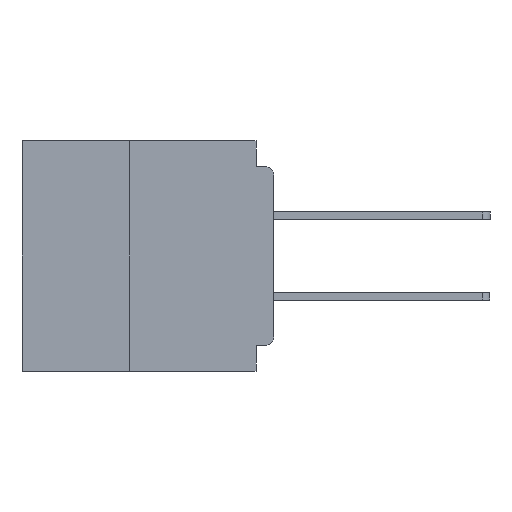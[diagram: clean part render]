
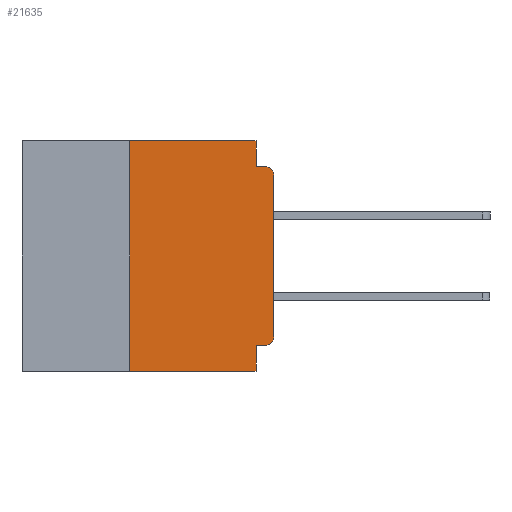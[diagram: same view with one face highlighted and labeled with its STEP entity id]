
A CAD part, left-side view. The second image highlights one B-rep face of the part: STEP entity #21635.
In plain terms, the highlighted planar face has unit normal (-1, 0, 0).
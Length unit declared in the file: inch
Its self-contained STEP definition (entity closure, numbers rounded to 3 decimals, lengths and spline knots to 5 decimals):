
#830 = CARTESIAN_POINT ( 'NONE',  ( 0., 0.031, 0. ) ) ;
#1980 = VECTOR ( 'NONE', #3878, 39.37008 ) ;
#3094 = ORIENTED_EDGE ( 'NONE', *, *, #14079, .T. ) ;
#3590 = DIRECTION ( 'NONE',  ( 0., -1., 0. ) ) ;
#3734 = VERTEX_POINT ( 'NONE', #43032 ) ;
#3878 = DIRECTION ( 'NONE',  ( 0., 0., 1. ) ) ;
#4229 = DIRECTION ( 'NONE',  ( 0., 0., -1. ) ) ;
#4340 = EDGE_LOOP ( 'NONE', ( #55539, #3094, #24114, #28395, #24261, #17673, #42425, #22083, #47247, #50970 ) ) ;
#7259 = VECTOR ( 'NONE', #3590, 39.37008 ) ;
#10152 = VERTEX_POINT ( 'NONE', #34538 ) ;
#10997 = LINE ( 'NONE', #52214, #56414 ) ;
#12163 = CARTESIAN_POINT ( 'NONE',  ( 0., 0.437, 0. ) ) ;
#13002 = VERTEX_POINT ( 'NONE', #40879 ) ;
#14079 = EDGE_CURVE ( 'NONE', #30475, #32978, #47007, .T. ) ;
#14602 = DIRECTION ( 'NONE',  ( 0., -1., 0. ) ) ;
#14851 = DIRECTION ( 'NONE',  ( 0., 0., -1. ) ) ;
#15622 = VECTOR ( 'NONE', #14602, 39.37008 ) ;
#15661 = DIRECTION ( 'NONE',  ( 0., 1., 0. ) ) ;
#15958 = EDGE_CURVE ( 'NONE', #10152, #30475, #38925, .T. ) ;
#17104 = VERTEX_POINT ( 'NONE', #26085 ) ;
#17262 = CARTESIAN_POINT ( 'NONE',  ( 0., 0., 0. ) ) ;
#17273 = DIRECTION ( 'NONE',  ( 0., 0., -1. ) ) ;
#17673 = ORIENTED_EDGE ( 'NONE', *, *, #23747, .F. ) ;
#17757 = EDGE_CURVE ( 'NONE', #3734, #13002, #10997, .T. ) ;
#19141 = CARTESIAN_POINT ( 'NONE',  ( 0., 0.437, -0.4 ) ) ;
#19378 = VERTEX_POINT ( 'NONE', #44471 ) ;
#20764 = EDGE_CURVE ( 'NONE', #30502, #13002, #28843, .T. ) ;
#21127 = VERTEX_POINT ( 'NONE', #43702 ) ;
#21635 = ADVANCED_FACE ( 'NONE', ( #37666 ), #57105, .F. ) ;
#22083 = ORIENTED_EDGE ( 'NONE', *, *, #17757, .F. ) ;
#22305 = CARTESIAN_POINT ( 'NONE',  ( 0., 0.25, -0.4 ) ) ;
#22745 = CARTESIAN_POINT ( 'NONE',  ( 0., 0.015, -0.34 ) ) ;
#23036 = VECTOR ( 'NONE', #38690, 39.37008 ) ;
#23747 = EDGE_CURVE ( 'NONE', #30502, #17104, #49830, .T. ) ;
#23801 = AXIS2_PLACEMENT_3D ( 'NONE', #22745, #53344, #27185 ) ;
#24005 = LINE ( 'NONE', #50662, #45956 ) ;
#24114 = ORIENTED_EDGE ( 'NONE', *, *, #49516, .F. ) ;
#24261 = ORIENTED_EDGE ( 'NONE', *, *, #52717, .F. ) ;
#25571 = AXIS2_PLACEMENT_3D ( 'NONE', #26553, #57095, #30978 ) ;
#25945 = CARTESIAN_POINT ( 'NONE',  ( 0., 0., -0.045 ) ) ;
#26085 = CARTESIAN_POINT ( 'NONE',  ( 0., 0.25, 0. ) ) ;
#26538 = VECTOR ( 'NONE', #40955, 39.37008 ) ;
#26553 = CARTESIAN_POINT ( 'NONE',  ( 0., 0.015, -0.06 ) ) ;
#27185 = DIRECTION ( 'NONE',  ( 0., 0., -1. ) ) ;
#28105 = CARTESIAN_POINT ( 'NONE',  ( 0., 0.031, 0. ) ) ;
#28395 = ORIENTED_EDGE ( 'NONE', *, *, #38484, .F. ) ;
#28843 = LINE ( 'NONE', #19141, #15622 ) ;
#28996 = EDGE_CURVE ( 'NONE', #19378, #3734, #24005, .T. ) ;
#29566 = LINE ( 'NONE', #25945, #7259 ) ;
#30475 = VERTEX_POINT ( 'NONE', #35217 ) ;
#30502 = VERTEX_POINT ( 'NONE', #22305 ) ;
#30524 = CARTESIAN_POINT ( 'NONE',  ( 0., 0.015, -0.045 ) ) ;
#30978 = DIRECTION ( 'NONE',  ( 0., 0., -1. ) ) ;
#30983 = DIRECTION ( 'NONE',  ( 1., 0., 0. ) ) ;
#31220 = CIRCLE ( 'NONE', #23801, 0.015 ) ;
#32068 = VECTOR ( 'NONE', #14851, 39.37008 ) ;
#32978 = VERTEX_POINT ( 'NONE', #30524 ) ;
#33473 = LINE ( 'NONE', #28105, #32068 ) ;
#34538 = CARTESIAN_POINT ( 'NONE',  ( 0., 0., -0.34 ) ) ;
#34750 = LINE ( 'NONE', #12163, #23036 ) ;
#35032 = CARTESIAN_POINT ( 'NONE',  ( 0., 0.437, 0. ) ) ;
#35217 = CARTESIAN_POINT ( 'NONE',  ( 0., 0., -0.06 ) ) ;
#36554 = CARTESIAN_POINT ( 'NONE',  ( 0., 0.25, -0.4 ) ) ;
#37666 = FACE_OUTER_BOUND ( 'NONE', #4340, .T. ) ;
#38484 = EDGE_CURVE ( 'NONE', #55324, #21127, #33473, .T. ) ;
#38690 = DIRECTION ( 'NONE',  ( 0., -1., 0. ) ) ;
#38925 = LINE ( 'NONE', #17262, #1980 ) ;
#40879 = CARTESIAN_POINT ( 'NONE',  ( 0., 0.031, -0.4 ) ) ;
#40955 = DIRECTION ( 'NONE',  ( 0., 0., 1. ) ) ;
#42425 = ORIENTED_EDGE ( 'NONE', *, *, #20764, .T. ) ;
#43032 = CARTESIAN_POINT ( 'NONE',  ( 0., 0.031, -0.355 ) ) ;
#43702 = CARTESIAN_POINT ( 'NONE',  ( 0., 0.031, -0.045 ) ) ;
#44471 = CARTESIAN_POINT ( 'NONE',  ( 0., 0.015, -0.355 ) ) ;
#45956 = VECTOR ( 'NONE', #15661, 39.37008 ) ;
#47007 = CIRCLE ( 'NONE', #25571, 0.015 ) ;
#47247 = ORIENTED_EDGE ( 'NONE', *, *, #28996, .F. ) ;
#49516 = EDGE_CURVE ( 'NONE', #21127, #32978, #29566, .T. ) ;
#49830 = LINE ( 'NONE', #36554, #26538 ) ;
#50662 = CARTESIAN_POINT ( 'NONE',  ( 0., 0., -0.355 ) ) ;
#50970 = ORIENTED_EDGE ( 'NONE', *, *, #53478, .T. ) ;
#52214 = CARTESIAN_POINT ( 'NONE',  ( 0., 0.031, -0.4 ) ) ;
#52717 = EDGE_CURVE ( 'NONE', #17104, #55324, #34750, .T. ) ;
#53344 = DIRECTION ( 'NONE',  ( -1., 0., 0. ) ) ;
#53478 = EDGE_CURVE ( 'NONE', #19378, #10152, #31220, .T. ) ;
#54250 = AXIS2_PLACEMENT_3D ( 'NONE', #35032, #30983, #4229 ) ;
#55324 = VERTEX_POINT ( 'NONE', #830 ) ;
#55539 = ORIENTED_EDGE ( 'NONE', *, *, #15958, .T. ) ;
#56414 = VECTOR ( 'NONE', #17273, 39.37008 ) ;
#57095 = DIRECTION ( 'NONE',  ( -1., 0., 0. ) ) ;
#57105 = PLANE ( 'NONE',  #54250 ) ;
